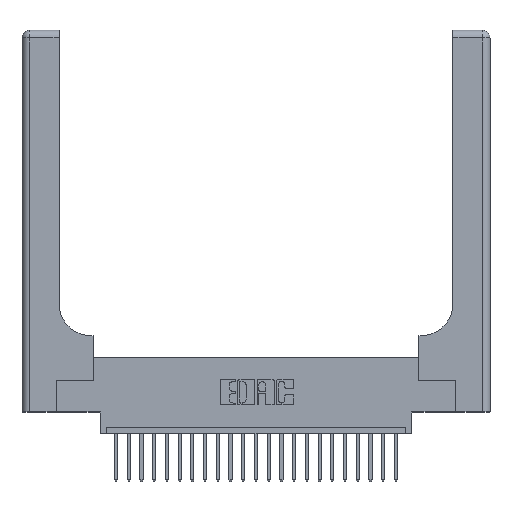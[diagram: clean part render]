
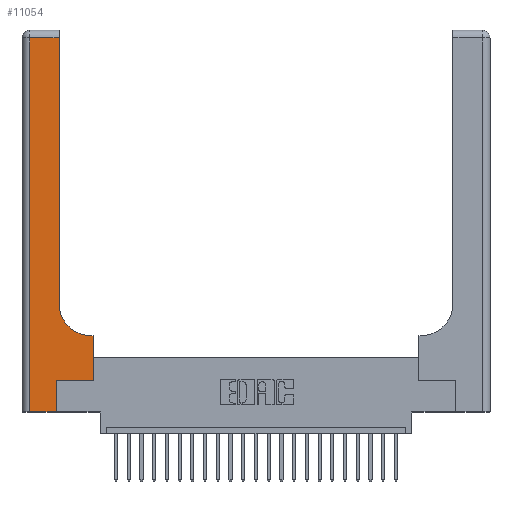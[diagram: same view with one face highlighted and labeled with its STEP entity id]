
A CAD part, top view. The second image highlights one B-rep face of the part: STEP entity #11054.
In plain terms, the highlighted planar face has unit normal (0, 0, 1).
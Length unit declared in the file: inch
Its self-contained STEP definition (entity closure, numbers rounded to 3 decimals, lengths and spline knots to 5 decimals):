
#78 = VECTOR ( 'NONE', #10641, 39.37008 ) ;
#150 = ORIENTED_EDGE ( 'NONE', *, *, #11952, .T. ) ;
#671 = DIRECTION ( 'NONE',  ( -1., 0., 0. ) ) ;
#806 = LINE ( 'NONE', #10835, #10583 ) ;
#1031 = EDGE_LOOP ( 'NONE', ( #150, #20115, #6988, #7709, #13204, #4300, #19700, #9165, #1709 ) ) ;
#1180 = CARTESIAN_POINT ( 'NONE',  ( 0., 2.94, 0.37 ) ) ;
#1709 = ORIENTED_EDGE ( 'NONE', *, *, #19539, .T. ) ;
#2174 = CARTESIAN_POINT ( 'NONE',  ( 0.5585, 0.25, 0.37 ) ) ;
#2433 = EDGE_CURVE ( 'NONE', #17103, #20808, #4437, .T. ) ;
#2881 = PLANE ( 'NONE',  #11578 ) ;
#2890 = CARTESIAN_POINT ( 'NONE',  ( 0.2915, 3., 0.37 ) ) ;
#4013 = VECTOR ( 'NONE', #18685, 39.37008 ) ;
#4300 = ORIENTED_EDGE ( 'NONE', *, *, #7434, .T. ) ;
#4437 = LINE ( 'NONE', #19450, #24516 ) ;
#4441 = EDGE_CURVE ( 'NONE', #11060, #13673, #806, .T. ) ;
#4845 = CARTESIAN_POINT ( 'NONE',  ( 0.269, 0.25, 0.37 ) ) ;
#5011 = FACE_OUTER_BOUND ( 'NONE', #1031, .T. ) ;
#6988 = ORIENTED_EDGE ( 'NONE', *, *, #2433, .T. ) ;
#7271 = CARTESIAN_POINT ( 'NONE',  ( 0.5415, 0.85, 0.37 ) ) ;
#7434 = EDGE_CURVE ( 'NONE', #15553, #11060, #20175, .T. ) ;
#7709 = ORIENTED_EDGE ( 'NONE', *, *, #11977, .T. ) ;
#8097 = DIRECTION ( 'NONE',  ( 0., -1., 0. ) ) ;
#8794 = CARTESIAN_POINT ( 'NONE',  ( 0., 0., 0.37 ) ) ;
#8923 = LINE ( 'NONE', #2890, #14670 ) ;
#9165 = ORIENTED_EDGE ( 'NONE', *, *, #16513, .T. ) ;
#10060 = VECTOR ( 'NONE', #14316, 39.37008 ) ;
#10141 = VECTOR ( 'NONE', #23982, 39.37008 ) ;
#10308 = CARTESIAN_POINT ( 'NONE',  ( 0.2915, 2.94, 0.37 ) ) ;
#10323 = CARTESIAN_POINT ( 'NONE',  ( 0., 3., 0.37 ) ) ;
#10404 = DIRECTION ( 'NONE',  ( 0., 0., -1. ) ) ;
#10583 = VECTOR ( 'NONE', #12506, 39.37008 ) ;
#10641 = DIRECTION ( 'NONE',  ( 1., 0., 0. ) ) ;
#10835 = CARTESIAN_POINT ( 'NONE',  ( 0.5585, 0.25, 0.37 ) ) ;
#11054 = ADVANCED_FACE ( 'NONE', ( #5011 ), #2881, .F. ) ;
#11060 = VERTEX_POINT ( 'NONE', #2174 ) ;
#11266 = DIRECTION ( 'NONE',  ( 0., 0., -1. ) ) ;
#11578 = AXIS2_PLACEMENT_3D ( 'NONE', #10323, #10404, #671 ) ;
#11843 = VECTOR ( 'NONE', #12066, 39.37008 ) ;
#11952 = EDGE_CURVE ( 'NONE', #22286, #20043, #8923, .T. ) ;
#11954 = LINE ( 'NONE', #8794, #10141 ) ;
#11977 = EDGE_CURVE ( 'NONE', #20808, #20931, #11954, .T. ) ;
#12066 = DIRECTION ( 'NONE',  ( 0., 1., 0. ) ) ;
#12506 = DIRECTION ( 'NONE',  ( 0., 1., 0. ) ) ;
#12934 = CARTESIAN_POINT ( 'NONE',  ( 0.06, 2.94, 0.37 ) ) ;
#12958 = AXIS2_PLACEMENT_3D ( 'NONE', #7271, #11266, #13017 ) ;
#13017 = DIRECTION ( 'NONE',  ( 1., 0., 0. ) ) ;
#13204 = ORIENTED_EDGE ( 'NONE', *, *, #20943, .T. ) ;
#13673 = VERTEX_POINT ( 'NONE', #18272 ) ;
#14316 = DIRECTION ( 'NONE',  ( -1., 0., 0. ) ) ;
#14670 = VECTOR ( 'NONE', #22141, 39.37008 ) ;
#15553 = VERTEX_POINT ( 'NONE', #20516 ) ;
#16513 = EDGE_CURVE ( 'NONE', #13673, #24126, #17594, .T. ) ;
#17103 = VERTEX_POINT ( 'NONE', #12934 ) ;
#17571 = CARTESIAN_POINT ( 'NONE',  ( 0.2915, 0.85, 0.37 ) ) ;
#17594 = LINE ( 'NONE', #24169, #10060 ) ;
#18173 = LINE ( 'NONE', #22011, #11843 ) ;
#18226 = CARTESIAN_POINT ( 'NONE',  ( 0.269, 0., 0.37 ) ) ;
#18272 = CARTESIAN_POINT ( 'NONE',  ( 0.5585, 0.6, 0.37 ) ) ;
#18685 = DIRECTION ( 'NONE',  ( -1., 0., 0. ) ) ;
#19450 = CARTESIAN_POINT ( 'NONE',  ( 0.06, 3., 0.37 ) ) ;
#19539 = EDGE_CURVE ( 'NONE', #24126, #22286, #23748, .T. ) ;
#19700 = ORIENTED_EDGE ( 'NONE', *, *, #4441, .T. ) ;
#19920 = CARTESIAN_POINT ( 'NONE',  ( 0.5415, 0.6, 0.37 ) ) ;
#20043 = VERTEX_POINT ( 'NONE', #10308 ) ;
#20115 = ORIENTED_EDGE ( 'NONE', *, *, #24973, .T. ) ;
#20175 = LINE ( 'NONE', #4845, #78 ) ;
#20516 = CARTESIAN_POINT ( 'NONE',  ( 0.269, 0.25, 0.37 ) ) ;
#20808 = VERTEX_POINT ( 'NONE', #23529 ) ;
#20931 = VERTEX_POINT ( 'NONE', #18226 ) ;
#20943 = EDGE_CURVE ( 'NONE', #20931, #15553, #18173, .T. ) ;
#22011 = CARTESIAN_POINT ( 'NONE',  ( 0.269, 0., 0.37 ) ) ;
#22141 = DIRECTION ( 'NONE',  ( 0., 1., 0. ) ) ;
#22286 = VERTEX_POINT ( 'NONE', #17571 ) ;
#23529 = CARTESIAN_POINT ( 'NONE',  ( 0.06, 0., 0.37 ) ) ;
#23748 = CIRCLE ( 'NONE', #12958, 0.25 ) ;
#23982 = DIRECTION ( 'NONE',  ( 1., 0., 0. ) ) ;
#24126 = VERTEX_POINT ( 'NONE', #19920 ) ;
#24169 = CARTESIAN_POINT ( 'NONE',  ( 0.2915, 0.6, 0.37 ) ) ;
#24516 = VECTOR ( 'NONE', #8097, 39.37008 ) ;
#24697 = LINE ( 'NONE', #1180, #4013 ) ;
#24973 = EDGE_CURVE ( 'NONE', #20043, #17103, #24697, .T. ) ;
